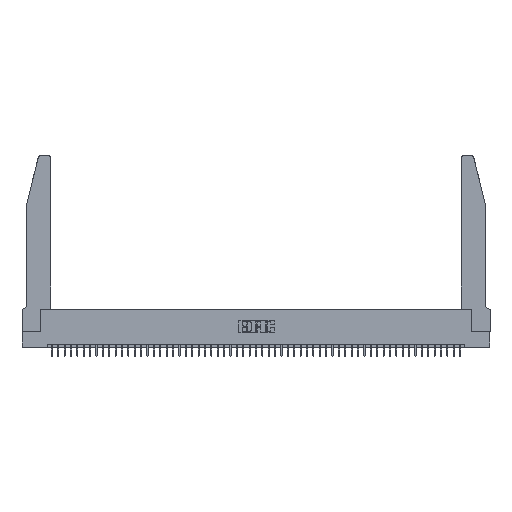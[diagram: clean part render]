
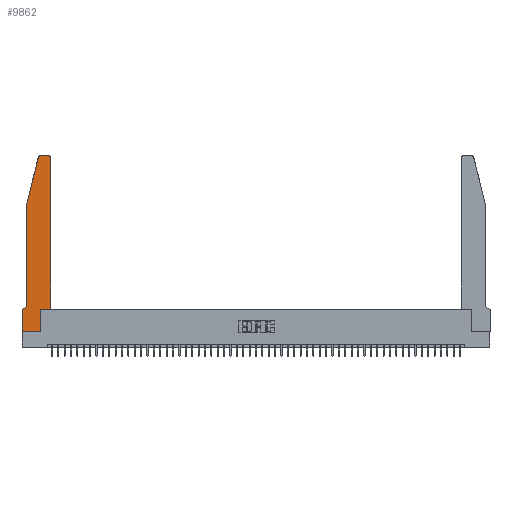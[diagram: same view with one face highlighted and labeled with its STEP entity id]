
A CAD part, top view. The second image highlights one B-rep face of the part: STEP entity #9862.
In plain terms, the highlighted planar face has unit normal (0, 0, 1).
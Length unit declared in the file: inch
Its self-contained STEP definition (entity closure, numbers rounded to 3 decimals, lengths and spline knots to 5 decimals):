
#553 = VERTEX_POINT ( 'NONE', #31145 ) ;
#1061 = DIRECTION ( 'NONE',  ( 1., 0., 0. ) ) ;
#2193 = DIRECTION ( 'NONE',  ( 0., 0., 1. ) ) ;
#2276 = VECTOR ( 'NONE', #1061, 39.37008 ) ;
#3615 = CARTESIAN_POINT ( 'NONE',  ( 0., 0.35, 0.37 ) ) ;
#5067 = CIRCLE ( 'NONE', #44319, 0.03 ) ;
#6306 = DIRECTION ( 'NONE',  ( 1., 0., 0. ) ) ;
#6344 = CARTESIAN_POINT ( 'NONE',  ( 0.2865, 0.35, 0.37 ) ) ;
#6662 = CARTESIAN_POINT ( 'NONE',  ( 0.4505, 0.35, 0.37 ) ) ;
#6711 = AXIS2_PLACEMENT_3D ( 'NONE', #27065, #35326, #22801 ) ;
#6975 = VERTEX_POINT ( 'NONE', #3615 ) ;
#7329 = DIRECTION ( 'NONE',  ( 0., 1., 0. ) ) ;
#7712 = VECTOR ( 'NONE', #42153, 39.37008 ) ;
#7872 = DIRECTION ( 'NONE',  ( -0.239, -0.971, 0. ) ) ;
#8376 = CARTESIAN_POINT ( 'NONE',  ( 0.0755, 0.42, 0.37 ) ) ;
#9773 = VERTEX_POINT ( 'NONE', #41858 ) ;
#9862 = ADVANCED_FACE ( 'NONE', ( #14342 ), #18341, .T. ) ;
#10425 = VERTEX_POINT ( 'NONE', #30205 ) ;
#10849 = EDGE_CURVE ( 'NONE', #10425, #31978, #32830, .T. ) ;
#11148 = CARTESIAN_POINT ( 'NONE',  ( 0.0755, 2., 0.37 ) ) ;
#13869 = EDGE_CURVE ( 'NONE', #6975, #27282, #15404, .T. ) ;
#13946 = VECTOR ( 'NONE', #41863, 39.37008 ) ;
#14342 = FACE_OUTER_BOUND ( 'NONE', #18988, .T. ) ;
#15023 = ORIENTED_EDGE ( 'NONE', *, *, #10849, .T. ) ;
#15076 = VECTOR ( 'NONE', #7329, 39.37008 ) ;
#15404 = LINE ( 'NONE', #35958, #50591 ) ;
#16514 = LINE ( 'NONE', #25593, #13946 ) ;
#17128 = ORIENTED_EDGE ( 'NONE', *, *, #51272, .T. ) ;
#17539 = CARTESIAN_POINT ( 'NONE',  ( 0.4205, 2.72, 0.37 ) ) ;
#18341 = PLANE ( 'NONE',  #46864 ) ;
#18529 = DIRECTION ( 'NONE',  ( 1., 0., 0. ) ) ;
#18929 = EDGE_CURVE ( 'NONE', #36406, #6975, #22807, .T. ) ;
#18988 = EDGE_LOOP ( 'NONE', ( #17128, #34743, #51773, #50506, #45785, #41823, #36144, #32284, #15023, #44361, #38188, #46610 ) ) ;
#20187 = CARTESIAN_POINT ( 'NONE',  ( 0.0755, 2., 0.37 ) ) ;
#20563 = LINE ( 'NONE', #35795, #50800 ) ;
#20807 = EDGE_CURVE ( 'NONE', #27282, #10425, #22218, .T. ) ;
#20847 = VECTOR ( 'NONE', #26800, 39.37008 ) ;
#21595 = CARTESIAN_POINT ( 'NONE',  ( 0.2865, 0.35, 0.37 ) ) ;
#21693 = DIRECTION ( 'NONE',  ( 1., 0., 0. ) ) ;
#22070 = EDGE_CURVE ( 'NONE', #35001, #41897, #20563, .T. ) ;
#22218 = LINE ( 'NONE', #43304, #47254 ) ;
#22799 = DIRECTION ( 'NONE',  ( 1., 0., 0. ) ) ;
#22801 = DIRECTION ( 'NONE',  ( -1., 0., 0. ) ) ;
#22807 = LINE ( 'NONE', #42806, #20847 ) ;
#23328 = EDGE_CURVE ( 'NONE', #35835, #553, #31647, .T. ) ;
#23447 = VERTEX_POINT ( 'NONE', #49246 ) ;
#23820 = EDGE_CURVE ( 'NONE', #31978, #35835, #33150, .T. ) ;
#23898 = CIRCLE ( 'NONE', #39245, 0.03 ) ;
#24237 = CARTESIAN_POINT ( 'NONE',  ( 0.0055, 0.35, 0.37 ) ) ;
#25593 = CARTESIAN_POINT ( 'NONE',  ( 0.2605, 2.75, 0.37 ) ) ;
#25703 = VERTEX_POINT ( 'NONE', #50437 ) ;
#26800 = DIRECTION ( 'NONE',  ( -1., 0., 0. ) ) ;
#27065 = CARTESIAN_POINT ( 'NONE',  ( 0.0055, 0.42, 0.37 ) ) ;
#27282 = VERTEX_POINT ( 'NONE', #51164 ) ;
#27593 = EDGE_CURVE ( 'NONE', #41897, #36406, #29753, .T. ) ;
#29056 = EDGE_CURVE ( 'NONE', #553, #25703, #23898, .T. ) ;
#29753 = CIRCLE ( 'NONE', #6711, 0.07 ) ;
#30205 = CARTESIAN_POINT ( 'NONE',  ( 0.2865, 0., 0.37 ) ) ;
#31145 = CARTESIAN_POINT ( 'NONE',  ( 0.4505, 2.72, 0.37 ) ) ;
#31647 = LINE ( 'NONE', #40706, #15076 ) ;
#31978 = VERTEX_POINT ( 'NONE', #21595 ) ;
#32284 = ORIENTED_EDGE ( 'NONE', *, *, #20807, .T. ) ;
#32830 = LINE ( 'NONE', #6344, #7712 ) ;
#33150 = LINE ( 'NONE', #45178, #2276 ) ;
#34743 = ORIENTED_EDGE ( 'NONE', *, *, #43317, .T. ) ;
#35001 = VERTEX_POINT ( 'NONE', #11148 ) ;
#35326 = DIRECTION ( 'NONE',  ( 0., 0., -1. ) ) ;
#35795 = CARTESIAN_POINT ( 'NONE',  ( 0.0755, 2., 0.37 ) ) ;
#35835 = VERTEX_POINT ( 'NONE', #6662 ) ;
#35958 = CARTESIAN_POINT ( 'NONE',  ( 0., 0., 0.37 ) ) ;
#36144 = ORIENTED_EDGE ( 'NONE', *, *, #13869, .T. ) ;
#36406 = VERTEX_POINT ( 'NONE', #24237 ) ;
#38188 = ORIENTED_EDGE ( 'NONE', *, *, #23328, .T. ) ;
#38305 = EDGE_CURVE ( 'NONE', #23447, #35001, #48501, .T. ) ;
#38527 = CARTESIAN_POINT ( 'NONE',  ( 0.284, 2.72, 0.37 ) ) ;
#39178 = CARTESIAN_POINT ( 'NONE',  ( 0., 0.35, 0.37 ) ) ;
#39245 = AXIS2_PLACEMENT_3D ( 'NONE', #17539, #42817, #18529 ) ;
#40593 = DIRECTION ( 'NONE',  ( 0., -1., 0. ) ) ;
#40706 = CARTESIAN_POINT ( 'NONE',  ( 0.4505, 0.35, 0.37 ) ) ;
#41328 = VECTOR ( 'NONE', #7872, 39.37008 ) ;
#41530 = DIRECTION ( 'NONE',  ( 0., -1., 0. ) ) ;
#41823 = ORIENTED_EDGE ( 'NONE', *, *, #18929, .T. ) ;
#41858 = CARTESIAN_POINT ( 'NONE',  ( 0.284, 2.75, 0.37 ) ) ;
#41863 = DIRECTION ( 'NONE',  ( -1., 0., 0. ) ) ;
#41897 = VERTEX_POINT ( 'NONE', #8376 ) ;
#42153 = DIRECTION ( 'NONE',  ( 0., 1., 0. ) ) ;
#42381 = DIRECTION ( 'NONE',  ( 0., 0., 1. ) ) ;
#42806 = CARTESIAN_POINT ( 'NONE',  ( 0.0755, 0.35, 0.37 ) ) ;
#42817 = DIRECTION ( 'NONE',  ( 0., 0., 1. ) ) ;
#43304 = CARTESIAN_POINT ( 'NONE',  ( 0., 0., 0.37 ) ) ;
#43317 = EDGE_CURVE ( 'NONE', #9773, #23447, #5067, .T. ) ;
#44319 = AXIS2_PLACEMENT_3D ( 'NONE', #38527, #2193, #22799 ) ;
#44361 = ORIENTED_EDGE ( 'NONE', *, *, #23820, .T. ) ;
#45178 = CARTESIAN_POINT ( 'NONE',  ( 0.4505, 0.35, 0.37 ) ) ;
#45785 = ORIENTED_EDGE ( 'NONE', *, *, #27593, .T. ) ;
#46610 = ORIENTED_EDGE ( 'NONE', *, *, #29056, .T. ) ;
#46864 = AXIS2_PLACEMENT_3D ( 'NONE', #39178, #42381, #6306 ) ;
#47254 = VECTOR ( 'NONE', #21693, 39.37008 ) ;
#48501 = LINE ( 'NONE', #20187, #41328 ) ;
#49246 = CARTESIAN_POINT ( 'NONE',  ( 0.25487, 2.72718, 0.37 ) ) ;
#50437 = CARTESIAN_POINT ( 'NONE',  ( 0.4205, 2.75, 0.37 ) ) ;
#50506 = ORIENTED_EDGE ( 'NONE', *, *, #22070, .T. ) ;
#50591 = VECTOR ( 'NONE', #41530, 39.37008 ) ;
#50800 = VECTOR ( 'NONE', #40593, 39.37008 ) ;
#51164 = CARTESIAN_POINT ( 'NONE',  ( 0., 0., 0.37 ) ) ;
#51272 = EDGE_CURVE ( 'NONE', #25703, #9773, #16514, .T. ) ;
#51773 = ORIENTED_EDGE ( 'NONE', *, *, #38305, .T. ) ;
